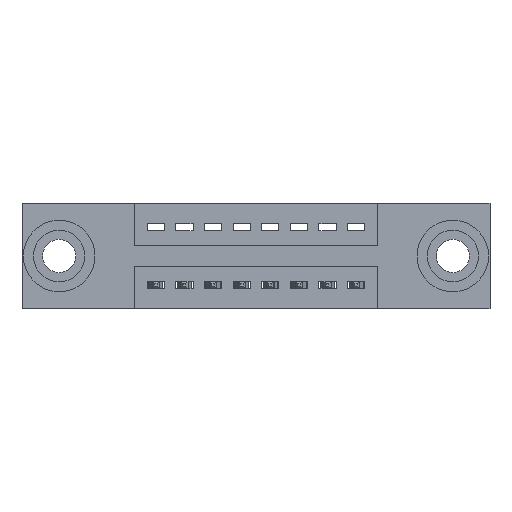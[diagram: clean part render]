
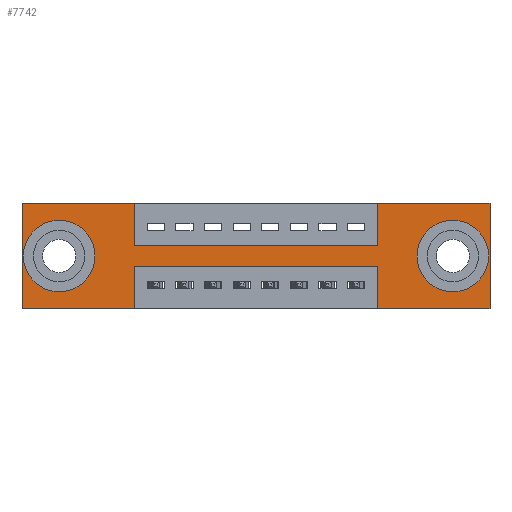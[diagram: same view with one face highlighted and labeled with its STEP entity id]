
A CAD part, front view. The second image highlights one B-rep face of the part: STEP entity #7742.
In plain terms, the highlighted planar face has unit normal (0, -1, 0).
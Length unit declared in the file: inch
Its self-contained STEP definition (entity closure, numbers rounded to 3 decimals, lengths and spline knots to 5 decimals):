
#7 = LINE ( 'NONE', #4737, #3928 ) ;
#89 = EDGE_CURVE ( 'NONE', #5232, #10015, #9795, .T. ) ;
#127 = VECTOR ( 'NONE', #4976, 39.37008 ) ;
#142 = EDGE_CURVE ( 'NONE', #6167, #467, #7, .T. ) ;
#319 = FACE_OUTER_BOUND ( 'NONE', #1104, .T. ) ;
#376 = VERTEX_POINT ( 'NONE', #4993 ) ;
#467 = VERTEX_POINT ( 'NONE', #6092 ) ;
#497 = VERTEX_POINT ( 'NONE', #4314 ) ;
#572 = DIRECTION ( 'NONE',  ( 0., -1., 0. ) ) ;
#573 = AXIS2_PLACEMENT_3D ( 'NONE', #5863, #11218, #7562 ) ;
#629 = CARTESIAN_POINT ( 'NONE',  ( 0.13, 0., -0.185 ) ) ;
#654 = CARTESIAN_POINT ( 'NONE',  ( 0.3925, 0., -0.22 ) ) ;
#665 = CARTESIAN_POINT ( 'NONE',  ( 0., 0., -0.37 ) ) ;
#723 = ORIENTED_EDGE ( 'NONE', *, *, #6720, .F. ) ;
#933 = EDGE_CURVE ( 'NONE', #4286, #6951, #5810, .T. ) ;
#981 = DIRECTION ( 'NONE',  ( 1., 0., 0. ) ) ;
#985 = VERTEX_POINT ( 'NONE', #4300 ) ;
#1090 = VECTOR ( 'NONE', #5382, 39.37008 ) ;
#1104 = EDGE_LOOP ( 'NONE', ( #6589, #8599, #10768, #2266, #3978, #3020, #10662, #4174, #1344, #2777, #723, #8096 ) ) ;
#1195 = VECTOR ( 'NONE', #10826, 39.37008 ) ;
#1215 = DIRECTION ( 'NONE',  ( 0., 0., -1. ) ) ;
#1234 = EDGE_CURVE ( 'NONE', #10015, #7778, #9775, .T. ) ;
#1344 = ORIENTED_EDGE ( 'NONE', *, *, #5712, .F. ) ;
#1363 = CARTESIAN_POINT ( 'NONE',  ( 1.2425, 0., -0.37 ) ) ;
#1444 = DIRECTION ( 'NONE',  ( 0., 0., 1. ) ) ;
#1515 = ORIENTED_EDGE ( 'NONE', *, *, #7450, .T. ) ;
#1672 = CARTESIAN_POINT ( 'NONE',  ( 0., 0., 0. ) ) ;
#1721 = AXIS2_PLACEMENT_3D ( 'NONE', #7152, #8915, #8070 ) ;
#1729 = CARTESIAN_POINT ( 'NONE',  ( 0.3925, 0., 0. ) ) ;
#1739 = CARTESIAN_POINT ( 'NONE',  ( 1.635, 0., 0. ) ) ;
#1894 = AXIS2_PLACEMENT_3D ( 'NONE', #6328, #8992, #1215 ) ;
#1923 = CARTESIAN_POINT ( 'NONE',  ( 0., 0., 0. ) ) ;
#2069 = CARTESIAN_POINT ( 'NONE',  ( 0., 0., 0. ) ) ;
#2238 = VERTEX_POINT ( 'NONE', #1672 ) ;
#2266 = ORIENTED_EDGE ( 'NONE', *, *, #89, .F. ) ;
#2280 = CARTESIAN_POINT ( 'NONE',  ( 0., 0., 0. ) ) ;
#2494 = LINE ( 'NONE', #2957, #11221 ) ;
#2527 = EDGE_CURVE ( 'NONE', #497, #985, #4303, .T. ) ;
#2544 = EDGE_CURVE ( 'NONE', #7975, #6981, #6056, .T. ) ;
#2604 = DIRECTION ( 'NONE',  ( 0., 0., -1. ) ) ;
#2662 = LINE ( 'NONE', #2280, #8903 ) ;
#2696 = CARTESIAN_POINT ( 'NONE',  ( 0.13, 0., -0.263 ) ) ;
#2777 = ORIENTED_EDGE ( 'NONE', *, *, #11287, .F. ) ;
#2846 = CARTESIAN_POINT ( 'NONE',  ( 1.2425, 0., -0.37 ) ) ;
#2957 = CARTESIAN_POINT ( 'NONE',  ( 0.3925, 0., -0.37 ) ) ;
#2994 = AXIS2_PLACEMENT_3D ( 'NONE', #8345, #572, #10081 ) ;
#3020 = ORIENTED_EDGE ( 'NONE', *, *, #2527, .F. ) ;
#3121 = VERTEX_POINT ( 'NONE', #11047 ) ;
#3259 = CARTESIAN_POINT ( 'NONE',  ( 0.3925, 0., -0.37 ) ) ;
#3364 = ORIENTED_EDGE ( 'NONE', *, *, #2544, .T. ) ;
#3443 = FACE_BOUND ( 'NONE', #10714, .T. ) ;
#3653 = CARTESIAN_POINT ( 'NONE',  ( 0.3925, 0., 0. ) ) ;
#3928 = VECTOR ( 'NONE', #5601, 39.37008 ) ;
#3978 = ORIENTED_EDGE ( 'NONE', *, *, #11072, .F. ) ;
#4061 = EDGE_CURVE ( 'NONE', #6981, #7975, #7891, .T. ) ;
#4079 = VECTOR ( 'NONE', #9578, 39.37008 ) ;
#4174 = ORIENTED_EDGE ( 'NONE', *, *, #142, .F. ) ;
#4253 = CARTESIAN_POINT ( 'NONE',  ( 0., 0., -0.37 ) ) ;
#4286 = VERTEX_POINT ( 'NONE', #3259 ) ;
#4300 = CARTESIAN_POINT ( 'NONE',  ( 1.635, 0., 0. ) ) ;
#4303 = LINE ( 'NONE', #1923, #11260 ) ;
#4314 = CARTESIAN_POINT ( 'NONE',  ( 1.2425, 0., 0. ) ) ;
#4357 = LINE ( 'NONE', #6931, #8293 ) ;
#4383 = AXIS2_PLACEMENT_3D ( 'NONE', #629, #10023, #6304 ) ;
#4737 = CARTESIAN_POINT ( 'NONE',  ( 0.3925, 0., -0.15 ) ) ;
#4831 = ORIENTED_EDGE ( 'NONE', *, *, #4061, .T. ) ;
#4938 = VERTEX_POINT ( 'NONE', #8431 ) ;
#4947 = EDGE_LOOP ( 'NONE', ( #4831, #3364 ) ) ;
#4968 = DIRECTION ( 'NONE',  ( -1., 0., 0. ) ) ;
#4976 = DIRECTION ( 'NONE',  ( -1., 0., 0. ) ) ;
#4993 = CARTESIAN_POINT ( 'NONE',  ( 1.505, 0., -0.263 ) ) ;
#5232 = VERTEX_POINT ( 'NONE', #8135 ) ;
#5329 = CARTESIAN_POINT ( 'NONE',  ( 0.3925, 0., -0.15 ) ) ;
#5364 = PLANE ( 'NONE',  #2994 ) ;
#5382 = DIRECTION ( 'NONE',  ( -1., 0., 0. ) ) ;
#5601 = DIRECTION ( 'NONE',  ( 1., 0., 0. ) ) ;
#5712 = EDGE_CURVE ( 'NONE', #9008, #6167, #8507, .T. ) ;
#5753 = CIRCLE ( 'NONE', #1894, 0.078 ) ;
#5810 = LINE ( 'NONE', #665, #127 ) ;
#5863 = CARTESIAN_POINT ( 'NONE',  ( 1.505, 0., -0.185 ) ) ;
#6018 = ORIENTED_EDGE ( 'NONE', *, *, #7106, .T. ) ;
#6056 = CIRCLE ( 'NONE', #4383, 0.078 ) ;
#6092 = CARTESIAN_POINT ( 'NONE',  ( 1.2425, 0., -0.15 ) ) ;
#6167 = VERTEX_POINT ( 'NONE', #5329 ) ;
#6286 = LINE ( 'NONE', #654, #7936 ) ;
#6292 = CARTESIAN_POINT ( 'NONE',  ( 0.13, 0., -0.107 ) ) ;
#6304 = DIRECTION ( 'NONE',  ( 0., 0., 1. ) ) ;
#6328 = CARTESIAN_POINT ( 'NONE',  ( 1.505, 0., -0.185 ) ) ;
#6519 = DIRECTION ( 'NONE',  ( 1., 0., 0. ) ) ;
#6576 = CARTESIAN_POINT ( 'NONE',  ( 1.2425, 0., -0.22 ) ) ;
#6589 = ORIENTED_EDGE ( 'NONE', *, *, #8282, .F. ) ;
#6720 = EDGE_CURVE ( 'NONE', #6951, #2238, #2662, .T. ) ;
#6931 = CARTESIAN_POINT ( 'NONE',  ( 1.2425, 0., 0. ) ) ;
#6951 = VERTEX_POINT ( 'NONE', #4253 ) ;
#6981 = VERTEX_POINT ( 'NONE', #6292 ) ;
#7066 = VECTOR ( 'NONE', #6519, 39.37008 ) ;
#7106 = EDGE_CURVE ( 'NONE', #376, #3121, #5753, .T. ) ;
#7152 = CARTESIAN_POINT ( 'NONE',  ( 0.13, 0., -0.185 ) ) ;
#7450 = EDGE_CURVE ( 'NONE', #3121, #376, #10689, .T. ) ;
#7562 = DIRECTION ( 'NONE',  ( 0., 0., -1. ) ) ;
#7742 = ADVANCED_FACE ( 'NONE', ( #3443, #9847, #319 ), #5364, .T. ) ;
#7778 = VERTEX_POINT ( 'NONE', #6576 ) ;
#7891 = CIRCLE ( 'NONE', #1721, 0.078 ) ;
#7900 = CARTESIAN_POINT ( 'NONE',  ( 0., 0., -0.37 ) ) ;
#7902 = EDGE_CURVE ( 'NONE', #7778, #4938, #6286, .T. ) ;
#7936 = VECTOR ( 'NONE', #4968, 39.37008 ) ;
#7975 = VERTEX_POINT ( 'NONE', #2696 ) ;
#8070 = DIRECTION ( 'NONE',  ( 0., 0., 1. ) ) ;
#8096 = ORIENTED_EDGE ( 'NONE', *, *, #933, .F. ) ;
#8135 = CARTESIAN_POINT ( 'NONE',  ( 1.635, 0., -0.37 ) ) ;
#8282 = EDGE_CURVE ( 'NONE', #4938, #4286, #2494, .T. ) ;
#8293 = VECTOR ( 'NONE', #9617, 39.37008 ) ;
#8345 = CARTESIAN_POINT ( 'NONE',  ( 0., 0., -0.37 ) ) ;
#8431 = CARTESIAN_POINT ( 'NONE',  ( 0.3925, 0., -0.22 ) ) ;
#8507 = LINE ( 'NONE', #1729, #10868 ) ;
#8599 = ORIENTED_EDGE ( 'NONE', *, *, #7902, .F. ) ;
#8903 = VECTOR ( 'NONE', #1444, 39.37008 ) ;
#8915 = DIRECTION ( 'NONE',  ( 0., 1., 0. ) ) ;
#8992 = DIRECTION ( 'NONE',  ( 0., 1., 0. ) ) ;
#9008 = VERTEX_POINT ( 'NONE', #3653 ) ;
#9144 = DIRECTION ( 'NONE',  ( 0., 0., -1. ) ) ;
#9578 = DIRECTION ( 'NONE',  ( 0., 0., -1. ) ) ;
#9617 = DIRECTION ( 'NONE',  ( 0., 0., 1. ) ) ;
#9775 = LINE ( 'NONE', #2846, #1195 ) ;
#9795 = LINE ( 'NONE', #7900, #1090 ) ;
#9847 = FACE_BOUND ( 'NONE', #4947, .T. ) ;
#10015 = VERTEX_POINT ( 'NONE', #1363 ) ;
#10023 = DIRECTION ( 'NONE',  ( 0., 1., 0. ) ) ;
#10081 = DIRECTION ( 'NONE',  ( 0., 0., -1. ) ) ;
#10230 = LINE ( 'NONE', #1739, #4079 ) ;
#10368 = LINE ( 'NONE', #2069, #7066 ) ;
#10662 = ORIENTED_EDGE ( 'NONE', *, *, #10953, .F. ) ;
#10689 = CIRCLE ( 'NONE', #573, 0.078 ) ;
#10714 = EDGE_LOOP ( 'NONE', ( #1515, #6018 ) ) ;
#10768 = ORIENTED_EDGE ( 'NONE', *, *, #1234, .F. ) ;
#10826 = DIRECTION ( 'NONE',  ( 0., 0., 1. ) ) ;
#10868 = VECTOR ( 'NONE', #2604, 39.37008 ) ;
#10953 = EDGE_CURVE ( 'NONE', #467, #497, #4357, .T. ) ;
#11047 = CARTESIAN_POINT ( 'NONE',  ( 1.505, 0., -0.107 ) ) ;
#11072 = EDGE_CURVE ( 'NONE', #985, #5232, #10230, .T. ) ;
#11218 = DIRECTION ( 'NONE',  ( 0., 1., 0. ) ) ;
#11221 = VECTOR ( 'NONE', #9144, 39.37008 ) ;
#11260 = VECTOR ( 'NONE', #981, 39.37008 ) ;
#11287 = EDGE_CURVE ( 'NONE', #2238, #9008, #10368, .T. ) ;
